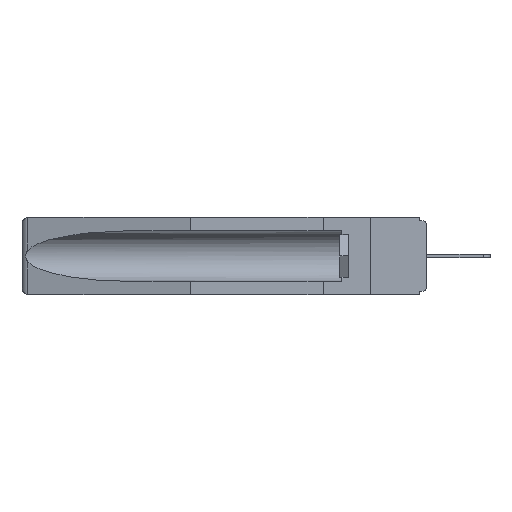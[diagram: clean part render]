
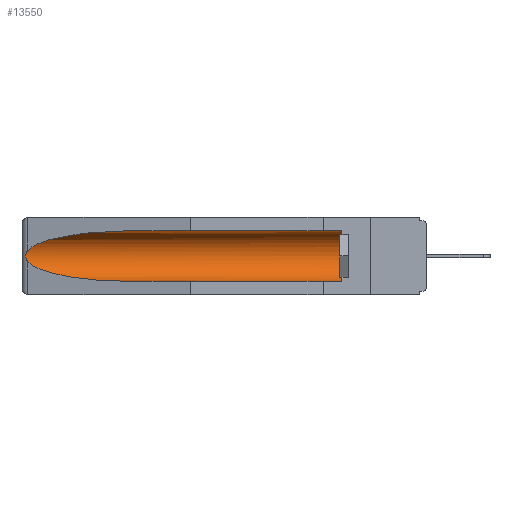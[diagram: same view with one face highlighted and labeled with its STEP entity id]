
A CAD part, left-side view. The second image highlights one B-rep face of the part: STEP entity #13550.
In plain terms, the highlighted cylindrical face has radius 2.857 mm (diameter 5.715 mm), a partial arc.
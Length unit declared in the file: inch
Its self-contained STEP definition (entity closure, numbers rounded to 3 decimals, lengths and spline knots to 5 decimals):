
#894 = ORIENTED_EDGE ( 'NONE', *, *, #4764, .T. ) ;
#1440 = VERTEX_POINT ( 'NONE', #19821 ) ;
#1817 = B_SPLINE_CURVE_WITH_KNOTS ( 'NONE', 3,
 ( #14747, #13045, #3540, #16693, #1824, #24020, #14513, #13169, #9388, #7573 ),
 .UNSPECIFIED., .F., .F.,
 ( 4, 2, 2, 2, 4 ),
 ( 0., 0.00029, 0.00058, 0.00087, 0.00117 ),
 .UNSPECIFIED. ) ;
#1824 = CARTESIAN_POINT ( 'NONE',  ( 0.2675, 1.53308, -0.16763 ) ) ;
#2154 = CARTESIAN_POINT ( 'NONE',  ( 0.155, 0.126, -0.059 ) ) ;
#2232 = EDGE_CURVE ( 'NONE', #1440, #10613, #11192, .T. ) ;
#2914 = CARTESIAN_POINT ( 'NONE',  ( 0.155, 0.126, -0.284 ) ) ;
#3261 = EDGE_CURVE ( 'NONE', #8230, #10613, #20020, .T. ) ;
#3540 = CARTESIAN_POINT ( 'NONE',  ( 0.26654, 1.53092, -0.15636 ) ) ;
#3990 = AXIS2_PLACEMENT_3D ( 'NONE', #22047, #22400, #9110 ) ;
#4055 = EDGE_LOOP ( 'NONE', ( #894, #20123, #9843, #16986, #15934, #11077 ) ) ;
#4203 = FACE_OUTER_BOUND ( 'NONE', #4055, .T. ) ;
#4475 = CARTESIAN_POINT ( 'NONE',  ( 0.155, 1.07973, -0.059 ) ) ;
#4764 = EDGE_CURVE ( 'NONE', #16551, #13711, #21164, .T. ) ;
#5860 = CARTESIAN_POINT ( 'NONE',  ( 0.25451, 1.48313, -0.24835 ) ) ;
#6818 = CARTESIAN_POINT ( 'NONE',  ( 0.155, 1.07973, -0.284 ) ) ;
#7573 = CARTESIAN_POINT ( 'NONE',  ( 0.26537, 1.52718, -0.19328 ) ) ;
#7824 = CARTESIAN_POINT ( 'NONE',  ( 0.21114, 1.30732, -0.059 ) ) ;
#8089 = DIRECTION ( 'NONE',  ( 0., 1., 0. ) ) ;
#8230 = VERTEX_POINT ( 'NONE', #2914 ) ;
#8380 = CARTESIAN_POINT ( 'NONE',  ( 0.155, 1.07973, -0.284 ) ) ;
#8440 = DIRECTION ( 'NONE',  ( 0., 1., 0. ) ) ;
#8675 = CARTESIAN_POINT ( 'NONE',  ( 0.26537, 1.52718, -0.14972 ) ) ;
#8702 = EDGE_CURVE ( 'NONE', #17671, #16551, #14208, .T. ) ;
#9110 = DIRECTION ( 'NONE',  ( 0., 0., 1. ) ) ;
#9388 = CARTESIAN_POINT ( 'NONE',  ( 0.26597, 1.5296, -0.19026 ) ) ;
#9433 = CIRCLE ( 'NONE', #3990, 0.1125 ) ;
#9843 = ORIENTED_EDGE ( 'NONE', *, *, #2232, .T. ) ;
#10613 = VERTEX_POINT ( 'NONE', #6818 ) ;
#11077 = ORIENTED_EDGE ( 'NONE', *, *, #8702, .T. ) ;
#11192 =( BOUNDED_CURVE ( )  B_SPLINE_CURVE ( 3, ( #17756, #5860, #18788, #8380 ),
 .UNSPECIFIED., .F., .F. ) 
 B_SPLINE_CURVE_WITH_KNOTS ( ( 4, 4 ),
 ( 0.1948, 1.5708 ),
 .UNSPECIFIED. ) 
 CURVE ( )  GEOMETRIC_REPRESENTATION_ITEM ( )  RATIONAL_B_SPLINE_CURVE ( ( 1., 0.848, 0.848, 1. ) ) 
 REPRESENTATION_ITEM ( '' )  );
#11635 = DIRECTION ( 'NONE',  ( 0., 0., 1. ) ) ;
#13045 = CARTESIAN_POINT ( 'NONE',  ( 0.26597, 1.52961, -0.15275 ) ) ;
#13169 = CARTESIAN_POINT ( 'NONE',  ( 0.26655, 1.53094, -0.18657 ) ) ;
#13550 = ADVANCED_FACE ( 'NONE', ( #4203 ), #13566, .F. ) ;
#13566 = CYLINDRICAL_SURFACE ( 'NONE', #16092, 0.1125 ) ;
#13711 = VERTEX_POINT ( 'NONE', #8675 ) ;
#14006 = VECTOR ( 'NONE', #14326, 39.37008 ) ;
#14208 = LINE ( 'NONE', #21668, #14006 ) ;
#14326 = DIRECTION ( 'NONE',  ( 0., 1., 0. ) ) ;
#14513 = CARTESIAN_POINT ( 'NONE',  ( 0.2673, 1.53269, -0.17917 ) ) ;
#14747 = CARTESIAN_POINT ( 'NONE',  ( 0.26537, 1.52718, -0.14972 ) ) ;
#15783 = EDGE_CURVE ( 'NONE', #13711, #1440, #1817, .T. ) ;
#15934 = ORIENTED_EDGE ( 'NONE', *, *, #22790, .T. ) ;
#16092 = AXIS2_PLACEMENT_3D ( 'NONE', #20896, #8089, #11635 ) ;
#16551 = VERTEX_POINT ( 'NONE', #4475 ) ;
#16693 = CARTESIAN_POINT ( 'NONE',  ( 0.2673, 1.5327, -0.16383 ) ) ;
#16986 = ORIENTED_EDGE ( 'NONE', *, *, #3261, .F. ) ;
#17671 = VERTEX_POINT ( 'NONE', #2154 ) ;
#17756 = CARTESIAN_POINT ( 'NONE',  ( 0.26537, 1.52718, -0.19328 ) ) ;
#18788 = CARTESIAN_POINT ( 'NONE',  ( 0.21114, 1.30732, -0.284 ) ) ;
#19155 = CARTESIAN_POINT ( 'NONE',  ( 0.26537, 1.52718, -0.14972 ) ) ;
#19534 = CARTESIAN_POINT ( 'NONE',  ( 0.155, -0.30754, -0.284 ) ) ;
#19821 = CARTESIAN_POINT ( 'NONE',  ( 0.26537, 1.52718, -0.19328 ) ) ;
#19914 = VECTOR ( 'NONE', #8440, 39.37008 ) ;
#20020 = LINE ( 'NONE', #19534, #19914 ) ;
#20123 = ORIENTED_EDGE ( 'NONE', *, *, #15783, .T. ) ;
#20896 = CARTESIAN_POINT ( 'NONE',  ( 0.155, -0.30754, -0.1715 ) ) ;
#21164 =( BOUNDED_CURVE ( )  B_SPLINE_CURVE ( 3, ( #23054, #7824, #21350, #19155 ),
 .UNSPECIFIED., .F., .F. ) 
 B_SPLINE_CURVE_WITH_KNOTS ( ( 4, 4 ),
 ( 4.71239, 6.08839 ),
 .UNSPECIFIED. ) 
 CURVE ( )  GEOMETRIC_REPRESENTATION_ITEM ( )  RATIONAL_B_SPLINE_CURVE ( ( 1., 0.848, 0.848, 1. ) ) 
 REPRESENTATION_ITEM ( '' )  );
#21350 = CARTESIAN_POINT ( 'NONE',  ( 0.25451, 1.48313, -0.09465 ) ) ;
#21668 = CARTESIAN_POINT ( 'NONE',  ( 0.155, -0.30754, -0.059 ) ) ;
#22047 = CARTESIAN_POINT ( 'NONE',  ( 0.155, 0.126, -0.1715 ) ) ;
#22400 = DIRECTION ( 'NONE',  ( 0., -1., 0. ) ) ;
#22790 = EDGE_CURVE ( 'NONE', #8230, #17671, #9433, .T. ) ;
#23054 = CARTESIAN_POINT ( 'NONE',  ( 0.155, 1.07973, -0.059 ) ) ;
#24020 = CARTESIAN_POINT ( 'NONE',  ( 0.2675, 1.53308, -0.17534 ) ) ;
